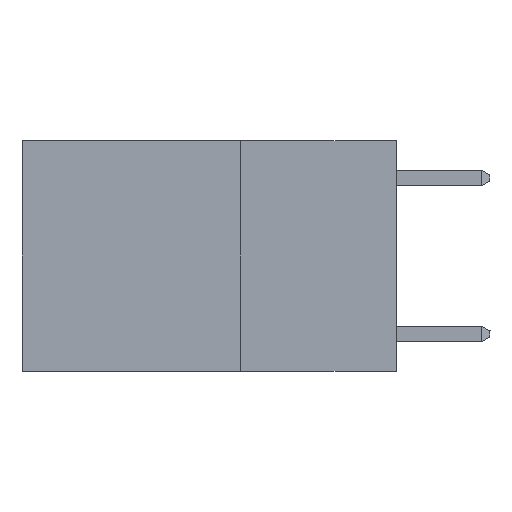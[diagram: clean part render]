
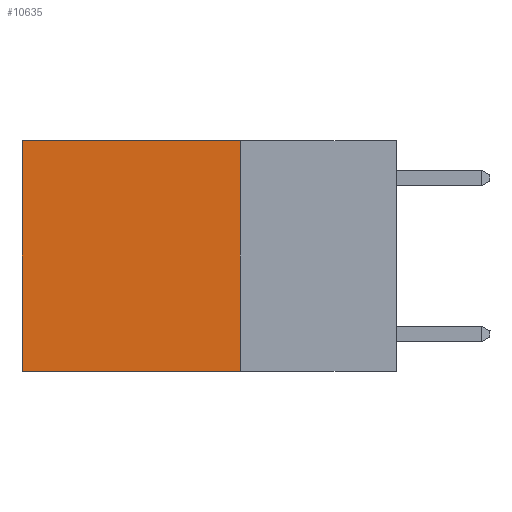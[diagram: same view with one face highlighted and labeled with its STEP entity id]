
A CAD part, left-side view. The second image highlights one B-rep face of the part: STEP entity #10635.
In plain terms, the highlighted planar face has unit normal (-1, 0, 0).
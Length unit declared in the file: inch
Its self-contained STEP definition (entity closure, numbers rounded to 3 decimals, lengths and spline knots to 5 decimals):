
#534 = ORIENTED_EDGE ( 'NONE', *, *, #29166, .F. ) ;
#1047 = CARTESIAN_POINT ( 'NONE',  ( 0.2625, 0.25, 0. ) ) ;
#1168 = ORIENTED_EDGE ( 'NONE', *, *, #29289, .T. ) ;
#4253 = LINE ( 'NONE', #6632, #22310 ) ;
#4711 = VECTOR ( 'NONE', #15206, 39.37008 ) ;
#4787 = ORIENTED_EDGE ( 'NONE', *, *, #28344, .F. ) ;
#4857 = DIRECTION ( 'NONE',  ( 0., 1., 0. ) ) ;
#4916 = PLANE ( 'NONE',  #10615 ) ;
#6601 = VERTEX_POINT ( 'NONE', #28612 ) ;
#6632 = CARTESIAN_POINT ( 'NONE',  ( 0.2625, 0.6, 0. ) ) ;
#7229 = DIRECTION ( 'NONE',  ( 1., 0., 0. ) ) ;
#7620 = VECTOR ( 'NONE', #14697, 39.37008 ) ;
#9001 = CARTESIAN_POINT ( 'NONE',  ( 0.2625, 0.25, 0. ) ) ;
#9561 = CARTESIAN_POINT ( 'NONE',  ( 0.2625, 0.25, -0.37 ) ) ;
#10615 = AXIS2_PLACEMENT_3D ( 'NONE', #28219, #7229, #23720 ) ;
#10635 = ADVANCED_FACE ( 'NONE', ( #13656 ), #4916, .F. ) ;
#10946 = LINE ( 'NONE', #1047, #4711 ) ;
#11597 = VERTEX_POINT ( 'NONE', #9001 ) ;
#11615 = ORIENTED_EDGE ( 'NONE', *, *, #21265, .T. ) ;
#11744 = LINE ( 'NONE', #9561, #18038 ) ;
#12413 = CARTESIAN_POINT ( 'NONE',  ( 0.2625, 0.25, 0. ) ) ;
#12796 = CARTESIAN_POINT ( 'NONE',  ( 0.2625, 0.6, -0.37 ) ) ;
#13656 = FACE_OUTER_BOUND ( 'NONE', #27761, .T. ) ;
#14697 = DIRECTION ( 'NONE',  ( 0., 0., -1. ) ) ;
#15206 = DIRECTION ( 'NONE',  ( 0., 1., 0. ) ) ;
#17835 = VERTEX_POINT ( 'NONE', #12796 ) ;
#18007 = VERTEX_POINT ( 'NONE', #23166 ) ;
#18038 = VECTOR ( 'NONE', #4857, 39.37008 ) ;
#20181 = LINE ( 'NONE', #12413, #7620 ) ;
#21265 = EDGE_CURVE ( 'NONE', #6601, #17835, #4253, .T. ) ;
#22310 = VECTOR ( 'NONE', #23096, 39.37008 ) ;
#23096 = DIRECTION ( 'NONE',  ( 0., 0., -1. ) ) ;
#23166 = CARTESIAN_POINT ( 'NONE',  ( 0.2625, 0.25, -0.37 ) ) ;
#23720 = DIRECTION ( 'NONE',  ( 0., 0., -1. ) ) ;
#27761 = EDGE_LOOP ( 'NONE', ( #11615, #4787, #534, #1168 ) ) ;
#28219 = CARTESIAN_POINT ( 'NONE',  ( 0.2625, 0.25, 0. ) ) ;
#28344 = EDGE_CURVE ( 'NONE', #18007, #17835, #11744, .T. ) ;
#28612 = CARTESIAN_POINT ( 'NONE',  ( 0.2625, 0.6, 0. ) ) ;
#29166 = EDGE_CURVE ( 'NONE', #11597, #18007, #20181, .T. ) ;
#29289 = EDGE_CURVE ( 'NONE', #11597, #6601, #10946, .T. ) ;
